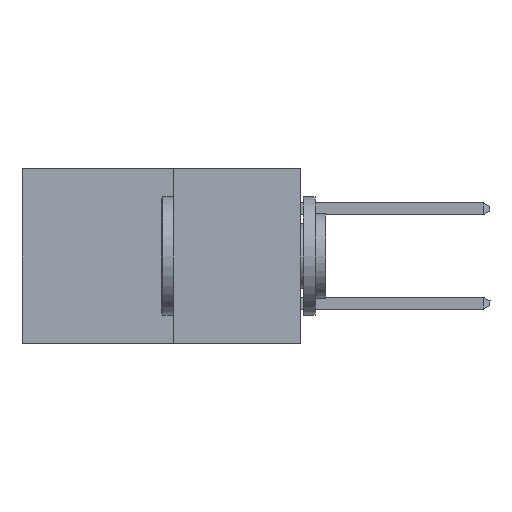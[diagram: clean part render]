
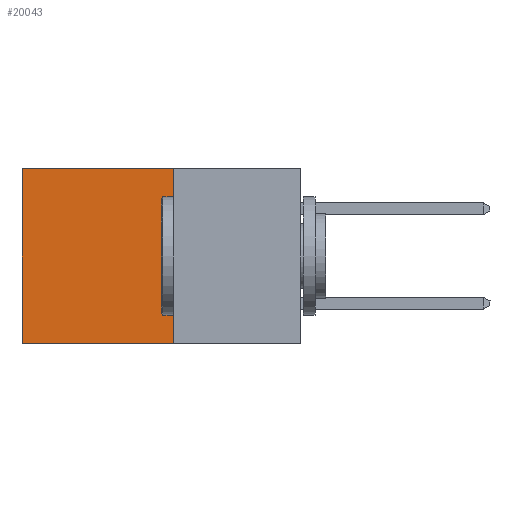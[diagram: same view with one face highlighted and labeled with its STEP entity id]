
A CAD part, left-side view. The second image highlights one B-rep face of the part: STEP entity #20043.
In plain terms, the highlighted planar face has unit normal (-1, 0, 0).
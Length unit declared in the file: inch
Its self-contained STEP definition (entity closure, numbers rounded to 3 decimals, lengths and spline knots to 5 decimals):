
#414 = LINE ( 'NONE', #13455, #9735 ) ;
#1428 = ORIENTED_EDGE ( 'NONE', *, *, #8806, .T. ) ;
#1631 = PLANE ( 'NONE',  #15743 ) ;
#1636 = ORIENTED_EDGE ( 'NONE', *, *, #4231, .F. ) ;
#2476 = VERTEX_POINT ( 'NONE', #15478 ) ;
#2755 = EDGE_CURVE ( 'NONE', #21831, #2476, #7110, .T. ) ;
#3097 = DIRECTION ( 'NONE',  ( 0., 1., 0. ) ) ;
#3403 = DIRECTION ( 'NONE',  ( 0., 0., -1. ) ) ;
#4231 = EDGE_CURVE ( 'NONE', #13705, #2476, #14550, .T. ) ;
#5945 = VECTOR ( 'NONE', #18514, 39.37008 ) ;
#6322 = ORIENTED_EDGE ( 'NONE', *, *, #19727, .F. ) ;
#7110 = LINE ( 'NONE', #10914, #20303 ) ;
#7721 = CARTESIAN_POINT ( 'NONE',  ( 0.277, 0.27, 0. ) ) ;
#7891 = ORIENTED_EDGE ( 'NONE', *, *, #2755, .T. ) ;
#8806 = EDGE_CURVE ( 'NONE', #15377, #21831, #414, .T. ) ;
#9618 = DIRECTION ( 'NONE',  ( 0., 0., -1. ) ) ;
#9735 = VECTOR ( 'NONE', #3097, 39.37008 ) ;
#10189 = FACE_OUTER_BOUND ( 'NONE', #16604, .T. ) ;
#10914 = CARTESIAN_POINT ( 'NONE',  ( 0.277, 0.59, -0.37 ) ) ;
#13013 = DIRECTION ( 'NONE',  ( 0., 0., -1. ) ) ;
#13455 = CARTESIAN_POINT ( 'NONE',  ( 0.277, 0.27, 0. ) ) ;
#13705 = VERTEX_POINT ( 'NONE', #20230 ) ;
#14550 = LINE ( 'NONE', #18998, #5945 ) ;
#14761 = CARTESIAN_POINT ( 'NONE',  ( 0.277, 0.27, -0.37 ) ) ;
#15377 = VERTEX_POINT ( 'NONE', #7721 ) ;
#15478 = CARTESIAN_POINT ( 'NONE',  ( 0.277, 0.59, -0.37 ) ) ;
#15743 = AXIS2_PLACEMENT_3D ( 'NONE', #22319, #17143, #3403 ) ;
#16109 = VECTOR ( 'NONE', #13013, 39.37008 ) ;
#16604 = EDGE_LOOP ( 'NONE', ( #7891, #1636, #6322, #1428 ) ) ;
#17143 = DIRECTION ( 'NONE',  ( 1., 0., 0. ) ) ;
#18514 = DIRECTION ( 'NONE',  ( 0., 1., 0. ) ) ;
#18998 = CARTESIAN_POINT ( 'NONE',  ( 0.277, 0.27, -0.37 ) ) ;
#19727 = EDGE_CURVE ( 'NONE', #15377, #13705, #21261, .T. ) ;
#20043 = ADVANCED_FACE ( 'NONE', ( #10189 ), #1631, .F. ) ;
#20230 = CARTESIAN_POINT ( 'NONE',  ( 0.277, 0.27, -0.37 ) ) ;
#20303 = VECTOR ( 'NONE', #9618, 39.37008 ) ;
#21261 = LINE ( 'NONE', #14761, #16109 ) ;
#21657 = CARTESIAN_POINT ( 'NONE',  ( 0.277, 0.59, 0. ) ) ;
#21831 = VERTEX_POINT ( 'NONE', #21657 ) ;
#22319 = CARTESIAN_POINT ( 'NONE',  ( 0.277, 0.27, -0.37 ) ) ;
